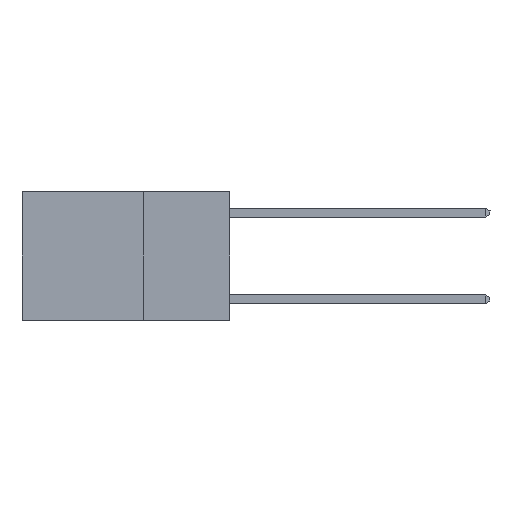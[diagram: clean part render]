
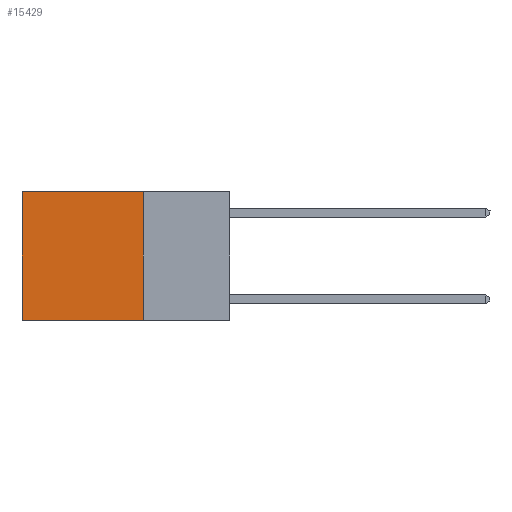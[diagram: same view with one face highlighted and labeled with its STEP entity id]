
A CAD part, left-side view. The second image highlights one B-rep face of the part: STEP entity #15429.
In plain terms, the highlighted planar face has unit normal (-1, 0, 0).
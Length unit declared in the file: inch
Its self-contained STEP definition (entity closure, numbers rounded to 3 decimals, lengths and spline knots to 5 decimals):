
#758 = ORIENTED_EDGE ( 'NONE', *, *, #4424, .F. ) ;
#903 = LINE ( 'NONE', #16980, #3674 ) ;
#1155 = VERTEX_POINT ( 'NONE', #4876 ) ;
#1518 = FACE_OUTER_BOUND ( 'NONE', #1623, .T. ) ;
#1623 = EDGE_LOOP ( 'NONE', ( #4228, #758, #17055, #5499 ) ) ;
#2016 = CARTESIAN_POINT ( 'NONE',  ( 0.2625, 0.25, 0. ) ) ;
#3226 = DIRECTION ( 'NONE',  ( 0., 0., -1. ) ) ;
#3389 = DIRECTION ( 'NONE',  ( 0., 0., -1. ) ) ;
#3674 = VECTOR ( 'NONE', #15678, 39.37008 ) ;
#4228 = ORIENTED_EDGE ( 'NONE', *, *, #7570, .T. ) ;
#4424 = EDGE_CURVE ( 'NONE', #7201, #1155, #903, .T. ) ;
#4509 = CARTESIAN_POINT ( 'NONE',  ( 0.2625, 0.25, 0. ) ) ;
#4805 = CARTESIAN_POINT ( 'NONE',  ( 0.2625, 0.25, 0. ) ) ;
#4876 = CARTESIAN_POINT ( 'NONE',  ( 0.2625, 0.6, -0.37 ) ) ;
#5499 = ORIENTED_EDGE ( 'NONE', *, *, #11286, .T. ) ;
#5837 = CARTESIAN_POINT ( 'NONE',  ( 0.2625, 0.6, 0. ) ) ;
#5878 = CARTESIAN_POINT ( 'NONE',  ( 0.2625, 0.25, 0. ) ) ;
#6172 = VERTEX_POINT ( 'NONE', #5837 ) ;
#7201 = VERTEX_POINT ( 'NONE', #11736 ) ;
#7570 = EDGE_CURVE ( 'NONE', #6172, #1155, #7633, .T. ) ;
#7633 = LINE ( 'NONE', #11167, #14456 ) ;
#8717 = AXIS2_PLACEMENT_3D ( 'NONE', #2016, #11330, #3389 ) ;
#8739 = PLANE ( 'NONE',  #8717 ) ;
#9848 = LINE ( 'NONE', #5878, #13231 ) ;
#10649 = LINE ( 'NONE', #4805, #13667 ) ;
#10832 = EDGE_CURVE ( 'NONE', #16037, #7201, #10649, .T. ) ;
#11167 = CARTESIAN_POINT ( 'NONE',  ( 0.2625, 0.6, 0. ) ) ;
#11286 = EDGE_CURVE ( 'NONE', #16037, #6172, #9848, .T. ) ;
#11330 = DIRECTION ( 'NONE',  ( 1., 0., 0. ) ) ;
#11373 = DIRECTION ( 'NONE',  ( 0., 0., -1. ) ) ;
#11736 = CARTESIAN_POINT ( 'NONE',  ( 0.2625, 0.25, -0.37 ) ) ;
#13231 = VECTOR ( 'NONE', #14992, 39.37008 ) ;
#13667 = VECTOR ( 'NONE', #11373, 39.37008 ) ;
#14456 = VECTOR ( 'NONE', #3226, 39.37008 ) ;
#14992 = DIRECTION ( 'NONE',  ( 0., 1., 0. ) ) ;
#15429 = ADVANCED_FACE ( 'NONE', ( #1518 ), #8739, .F. ) ;
#15678 = DIRECTION ( 'NONE',  ( 0., 1., 0. ) ) ;
#16037 = VERTEX_POINT ( 'NONE', #4509 ) ;
#16980 = CARTESIAN_POINT ( 'NONE',  ( 0.2625, 0.25, -0.37 ) ) ;
#17055 = ORIENTED_EDGE ( 'NONE', *, *, #10832, .F. ) ;
